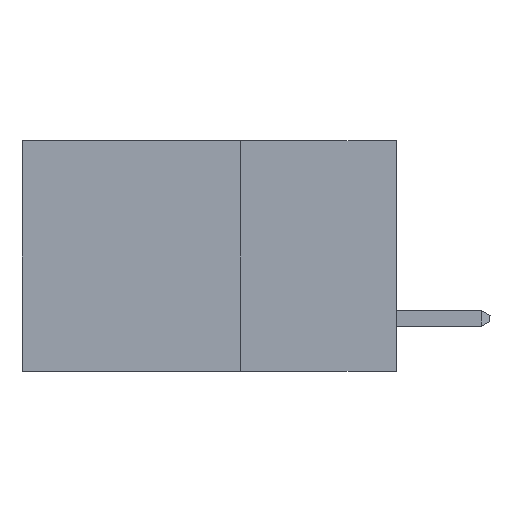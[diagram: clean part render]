
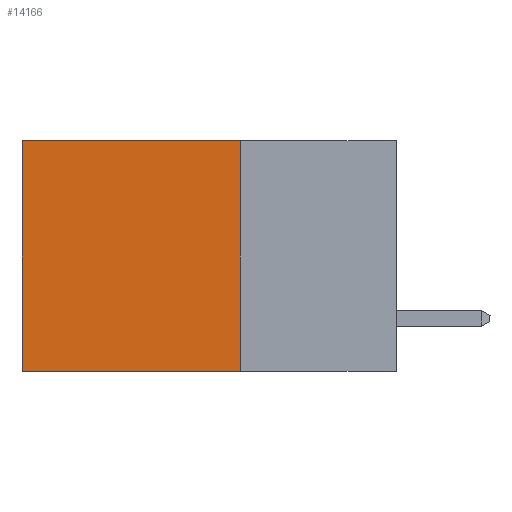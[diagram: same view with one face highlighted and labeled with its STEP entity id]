
A CAD part, left-side view. The second image highlights one B-rep face of the part: STEP entity #14166.
In plain terms, the highlighted planar face has unit normal (-1, 0, 0).
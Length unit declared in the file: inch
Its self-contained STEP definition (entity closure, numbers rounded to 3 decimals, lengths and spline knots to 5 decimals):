
#378 = ORIENTED_EDGE ( 'NONE', *, *, #10776, .F. ) ;
#430 = EDGE_CURVE ( 'NONE', #10359, #16033, #3959, .T. ) ;
#3138 = LINE ( 'NONE', #17089, #6446 ) ;
#3870 = EDGE_CURVE ( 'NONE', #16033, #8560, #3138, .T. ) ;
#3959 = LINE ( 'NONE', #11911, #11744 ) ;
#4426 = ORIENTED_EDGE ( 'NONE', *, *, #3870, .T. ) ;
#4638 = VERTEX_POINT ( 'NONE', #5723 ) ;
#5011 = DIRECTION ( 'NONE',  ( 1., 0., 0. ) ) ;
#5723 = CARTESIAN_POINT ( 'NONE',  ( 0.2615, 0.25, -0.37 ) ) ;
#6446 = VECTOR ( 'NONE', #8753, 39.37008 ) ;
#7381 = CARTESIAN_POINT ( 'NONE',  ( 0.2615, 0.25, -0.37 ) ) ;
#8499 = AXIS2_PLACEMENT_3D ( 'NONE', #9160, #5011, #14632 ) ;
#8560 = VERTEX_POINT ( 'NONE', #10353 ) ;
#8753 = DIRECTION ( 'NONE',  ( 0., 0., -1. ) ) ;
#8816 = DIRECTION ( 'NONE',  ( 0., 0., -1. ) ) ;
#8972 = CARTESIAN_POINT ( 'NONE',  ( 0.2615, 0.25, -0.37 ) ) ;
#9160 = CARTESIAN_POINT ( 'NONE',  ( 0.2615, 0.25, -0.37 ) ) ;
#9424 = CARTESIAN_POINT ( 'NONE',  ( 0.2615, 0.25, 0. ) ) ;
#10353 = CARTESIAN_POINT ( 'NONE',  ( 0.2615, 0.6, -0.37 ) ) ;
#10359 = VERTEX_POINT ( 'NONE', #9424 ) ;
#10429 = LINE ( 'NONE', #7381, #13608 ) ;
#10776 = EDGE_CURVE ( 'NONE', #4638, #8560, #13691, .T. ) ;
#11041 = CARTESIAN_POINT ( 'NONE',  ( 0.2615, 0.6, 0. ) ) ;
#11489 = ORIENTED_EDGE ( 'NONE', *, *, #14001, .F. ) ;
#11744 = VECTOR ( 'NONE', #12317, 39.37008 ) ;
#11911 = CARTESIAN_POINT ( 'NONE',  ( 0.2615, 0.25, 0. ) ) ;
#12074 = ORIENTED_EDGE ( 'NONE', *, *, #430, .T. ) ;
#12317 = DIRECTION ( 'NONE',  ( 0., 1., 0. ) ) ;
#13063 = DIRECTION ( 'NONE',  ( 0., 1., 0. ) ) ;
#13255 = PLANE ( 'NONE',  #8499 ) ;
#13608 = VECTOR ( 'NONE', #8816, 39.37008 ) ;
#13691 = LINE ( 'NONE', #8972, #16870 ) ;
#14001 = EDGE_CURVE ( 'NONE', #10359, #4638, #10429, .T. ) ;
#14166 = ADVANCED_FACE ( 'NONE', ( #14229 ), #13255, .F. ) ;
#14229 = FACE_OUTER_BOUND ( 'NONE', #14423, .T. ) ;
#14423 = EDGE_LOOP ( 'NONE', ( #4426, #378, #11489, #12074 ) ) ;
#14632 = DIRECTION ( 'NONE',  ( 0., 0., -1. ) ) ;
#16033 = VERTEX_POINT ( 'NONE', #11041 ) ;
#16870 = VECTOR ( 'NONE', #13063, 39.37008 ) ;
#17089 = CARTESIAN_POINT ( 'NONE',  ( 0.2615, 0.6, -0.37 ) ) ;
